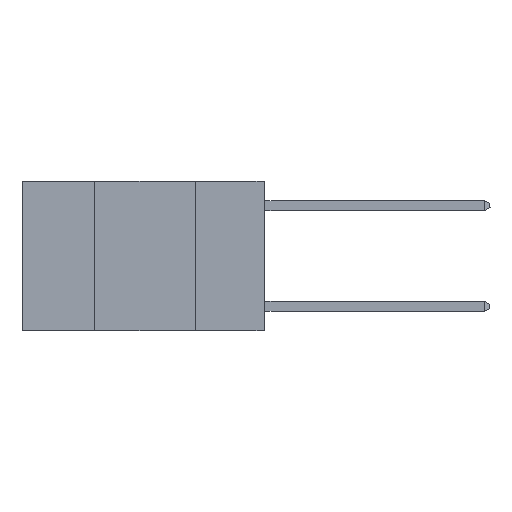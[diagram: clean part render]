
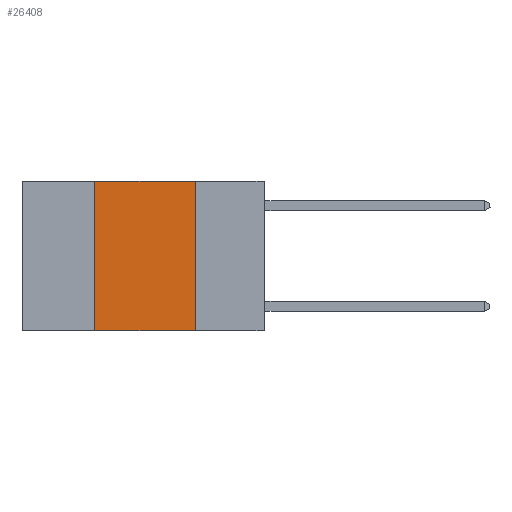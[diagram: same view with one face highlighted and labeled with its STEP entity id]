
A CAD part, left-side view. The second image highlights one B-rep face of the part: STEP entity #26408.
In plain terms, the highlighted planar face has unit normal (-1, 0, 0).
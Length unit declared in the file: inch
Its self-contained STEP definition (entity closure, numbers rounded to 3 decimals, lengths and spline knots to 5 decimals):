
#33 = EDGE_CURVE ( 'NONE', #26384, #2646, #24860, .T. ) ;
#220 = VECTOR ( 'NONE', #11950, 39.37008 ) ;
#775 = VECTOR ( 'NONE', #24136, 39.37008 ) ;
#1258 = CARTESIAN_POINT ( 'NONE',  ( 0., 0.6, 0. ) ) ;
#1546 = VECTOR ( 'NONE', #10354, 39.37008 ) ;
#1999 = DIRECTION ( 'NONE',  ( 0., 0., -1. ) ) ;
#2049 = PLANE ( 'NONE',  #2516 ) ;
#2516 = AXIS2_PLACEMENT_3D ( 'NONE', #24607, #8933, #24706 ) ;
#2646 = VERTEX_POINT ( 'NONE', #5965 ) ;
#3109 = EDGE_CURVE ( 'NONE', #26384, #5607, #25039, .T. ) ;
#3176 = FACE_OUTER_BOUND ( 'NONE', #28969, .T. ) ;
#3385 = CARTESIAN_POINT ( 'NONE',  ( 0., 0.17, 0. ) ) ;
#3598 = ORIENTED_EDGE ( 'NONE', *, *, #33, .T. ) ;
#5607 = VERTEX_POINT ( 'NONE', #13775 ) ;
#5965 = CARTESIAN_POINT ( 'NONE',  ( 0., 0.17, -0.37 ) ) ;
#6129 = VECTOR ( 'NONE', #1999, 39.37008 ) ;
#8226 = ORIENTED_EDGE ( 'NONE', *, *, #24908, .F. ) ;
#8933 = DIRECTION ( 'NONE',  ( 1., 0., 0. ) ) ;
#10354 = DIRECTION ( 'NONE',  ( 0., -1., 0. ) ) ;
#11950 = DIRECTION ( 'NONE',  ( 0., 0., 1. ) ) ;
#12044 = CARTESIAN_POINT ( 'NONE',  ( 0., 0.42, 0. ) ) ;
#12213 = LINE ( 'NONE', #28974, #6129 ) ;
#13775 = CARTESIAN_POINT ( 'NONE',  ( 0., 0.42, 0. ) ) ;
#19625 = LINE ( 'NONE', #1258, #1546 ) ;
#20086 = CARTESIAN_POINT ( 'NONE',  ( 0., 0.42, -0.37 ) ) ;
#20236 = ORIENTED_EDGE ( 'NONE', *, *, #23993, .F. ) ;
#20932 = ORIENTED_EDGE ( 'NONE', *, *, #3109, .F. ) ;
#21396 = VERTEX_POINT ( 'NONE', #3385 ) ;
#23993 = EDGE_CURVE ( 'NONE', #5607, #21396, #19625, .T. ) ;
#24136 = DIRECTION ( 'NONE',  ( 0., -1., 0. ) ) ;
#24607 = CARTESIAN_POINT ( 'NONE',  ( 0., 0.6, 0. ) ) ;
#24706 = DIRECTION ( 'NONE',  ( 0., 0., -1. ) ) ;
#24860 = LINE ( 'NONE', #26497, #775 ) ;
#24908 = EDGE_CURVE ( 'NONE', #21396, #2646, #12213, .T. ) ;
#25039 = LINE ( 'NONE', #12044, #220 ) ;
#26384 = VERTEX_POINT ( 'NONE', #20086 ) ;
#26408 = ADVANCED_FACE ( 'NONE', ( #3176 ), #2049, .F. ) ;
#26497 = CARTESIAN_POINT ( 'NONE',  ( 0., 0.6, -0.37 ) ) ;
#28969 = EDGE_LOOP ( 'NONE', ( #8226, #20236, #20932, #3598 ) ) ;
#28974 = CARTESIAN_POINT ( 'NONE',  ( 0., 0.17, 0. ) ) ;
